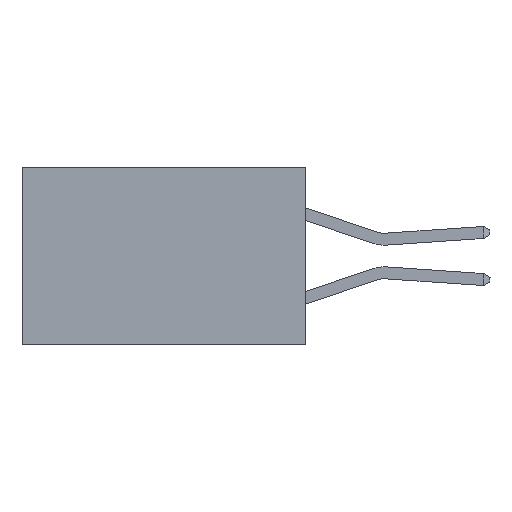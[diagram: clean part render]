
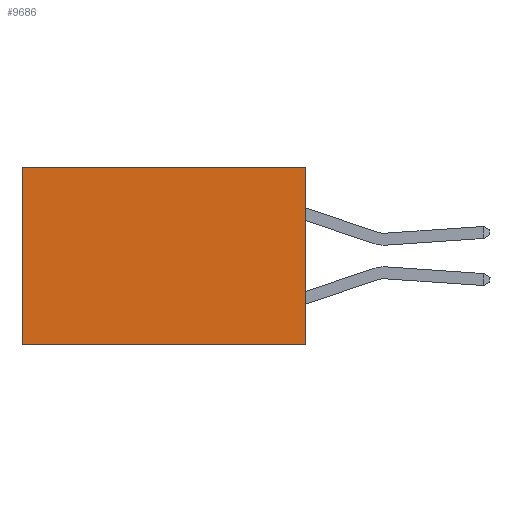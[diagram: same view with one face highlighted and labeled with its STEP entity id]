
A CAD part, left-side view. The second image highlights one B-rep face of the part: STEP entity #9686.
In plain terms, the highlighted planar face has unit normal (-1, 0, 0).
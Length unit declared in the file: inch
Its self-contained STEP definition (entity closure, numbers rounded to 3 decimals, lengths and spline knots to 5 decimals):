
#216 = ORIENTED_EDGE ( 'NONE', *, *, #14603, .F. ) ;
#1078 = DIRECTION ( 'NONE',  ( 0., 0., -1. ) ) ;
#3503 = DIRECTION ( 'NONE',  ( 0., 1., 0. ) ) ;
#3556 = CARTESIAN_POINT ( 'NONE',  ( 0.277, 0., 0. ) ) ;
#4578 = DIRECTION ( 'NONE',  ( 0., 1., 0. ) ) ;
#4716 = LINE ( 'NONE', #15371, #18399 ) ;
#5315 = EDGE_LOOP ( 'NONE', ( #21269, #9129, #216, #19446 ) ) ;
#5349 = CARTESIAN_POINT ( 'NONE',  ( 0.277, 0., -0.37 ) ) ;
#5828 = CARTESIAN_POINT ( 'NONE',  ( 0.277, 0.59, 0. ) ) ;
#6786 = VECTOR ( 'NONE', #3503, 39.37008 ) ;
#7349 = VERTEX_POINT ( 'NONE', #13380 ) ;
#7589 = VERTEX_POINT ( 'NONE', #11238 ) ;
#7987 = LINE ( 'NONE', #15516, #18440 ) ;
#8245 = CARTESIAN_POINT ( 'NONE',  ( 0.277, 0., -0.37 ) ) ;
#8373 = FACE_OUTER_BOUND ( 'NONE', #5315, .T. ) ;
#8400 = EDGE_CURVE ( 'NONE', #18523, #16191, #17342, .T. ) ;
#9129 = ORIENTED_EDGE ( 'NONE', *, *, #10072, .F. ) ;
#9182 = EDGE_CURVE ( 'NONE', #16191, #7589, #7987, .T. ) ;
#9202 = PLANE ( 'NONE',  #17935 ) ;
#9686 = ADVANCED_FACE ( 'NONE', ( #8373 ), #9202, .F. ) ;
#10072 = EDGE_CURVE ( 'NONE', #7349, #7589, #4716, .T. ) ;
#11238 = CARTESIAN_POINT ( 'NONE',  ( 0.277, 0.59, -0.37 ) ) ;
#12214 = LINE ( 'NONE', #5349, #17509 ) ;
#13380 = CARTESIAN_POINT ( 'NONE',  ( 0.277, 0., -0.37 ) ) ;
#13808 = DIRECTION ( 'NONE',  ( 0., 0., -1. ) ) ;
#14288 = DIRECTION ( 'NONE',  ( 1., 0., 0. ) ) ;
#14603 = EDGE_CURVE ( 'NONE', #18523, #7349, #12214, .T. ) ;
#15371 = CARTESIAN_POINT ( 'NONE',  ( 0.277, 0., -0.37 ) ) ;
#15516 = CARTESIAN_POINT ( 'NONE',  ( 0.277, 0.59, -0.37 ) ) ;
#16191 = VERTEX_POINT ( 'NONE', #5828 ) ;
#17342 = LINE ( 'NONE', #3556, #6786 ) ;
#17509 = VECTOR ( 'NONE', #17820, 39.37008 ) ;
#17820 = DIRECTION ( 'NONE',  ( 0., 0., -1. ) ) ;
#17935 = AXIS2_PLACEMENT_3D ( 'NONE', #8245, #14288, #13808 ) ;
#18399 = VECTOR ( 'NONE', #4578, 39.37008 ) ;
#18440 = VECTOR ( 'NONE', #1078, 39.37008 ) ;
#18523 = VERTEX_POINT ( 'NONE', #21628 ) ;
#19446 = ORIENTED_EDGE ( 'NONE', *, *, #8400, .T. ) ;
#21269 = ORIENTED_EDGE ( 'NONE', *, *, #9182, .T. ) ;
#21628 = CARTESIAN_POINT ( 'NONE',  ( 0.277, 0., 0. ) ) ;
